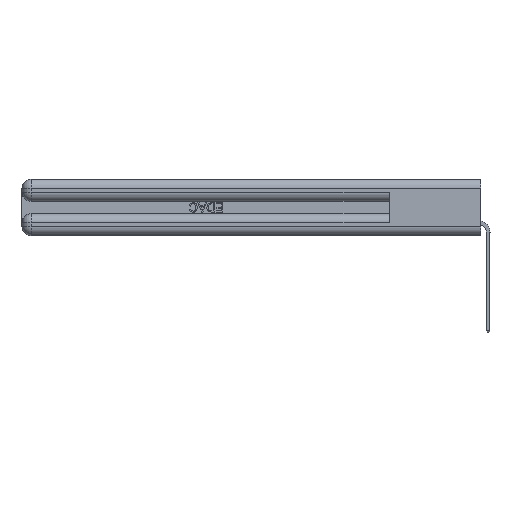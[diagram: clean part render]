
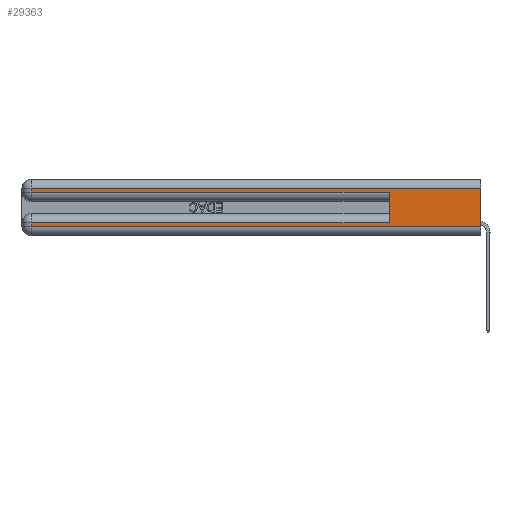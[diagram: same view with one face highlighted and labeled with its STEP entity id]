
A CAD part, left-side view. The second image highlights one B-rep face of the part: STEP entity #29363.
In plain terms, the highlighted planar face has unit normal (-1, 0, 0).
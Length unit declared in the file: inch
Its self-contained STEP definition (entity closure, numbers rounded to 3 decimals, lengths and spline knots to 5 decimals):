
#166 = DIRECTION ( 'NONE',  ( 0., 0., -1. ) ) ;
#222 = LINE ( 'NONE', #45272, #41382 ) ;
#773 = VECTOR ( 'NONE', #12997, 39.37008 ) ;
#2740 = EDGE_CURVE ( 'NONE', #19187, #14937, #31027, .T. ) ;
#3002 = EDGE_CURVE ( 'NONE', #6800, #37863, #222, .T. ) ;
#4448 = EDGE_CURVE ( 'NONE', #21822, #43918, #17563, .T. ) ;
#5373 = CARTESIAN_POINT ( 'NONE',  ( 0., 0., 0.31 ) ) ;
#5494 = PLANE ( 'NONE',  #32979 ) ;
#6591 = EDGE_CURVE ( 'NONE', #19187, #43918, #25633, .T. ) ;
#6682 = CARTESIAN_POINT ( 'NONE',  ( 0., 0.6, 0.145 ) ) ;
#6800 = VERTEX_POINT ( 'NONE', #9435 ) ;
#7109 = VECTOR ( 'NONE', #36315, 39.37008 ) ;
#7800 = VERTEX_POINT ( 'NONE', #29894 ) ;
#8801 = CARTESIAN_POINT ( 'NONE',  ( 0., 0., 0.37 ) ) ;
#9435 = CARTESIAN_POINT ( 'NONE',  ( 0., 2.94, 0.06 ) ) ;
#12997 = DIRECTION ( 'NONE',  ( 0., 0., -1. ) ) ;
#13910 = ORIENTED_EDGE ( 'NONE', *, *, #3002, .T. ) ;
#14516 = EDGE_CURVE ( 'NONE', #28528, #37863, #21750, .T. ) ;
#14787 = LINE ( 'NONE', #16875, #773 ) ;
#14937 = VERTEX_POINT ( 'NONE', #30757 ) ;
#15984 = VECTOR ( 'NONE', #29504, 39.37008 ) ;
#16369 = DIRECTION ( 'NONE',  ( 0., 0., -1. ) ) ;
#16875 = CARTESIAN_POINT ( 'NONE',  ( 0., 2.94, 0.37 ) ) ;
#17563 = LINE ( 'NONE', #45735, #30797 ) ;
#17865 = LINE ( 'NONE', #5373, #29418 ) ;
#19159 = DIRECTION ( 'NONE',  ( 0., 0., -1. ) ) ;
#19187 = VERTEX_POINT ( 'NONE', #41642 ) ;
#20234 = DIRECTION ( 'NONE',  ( 1., 0., 0. ) ) ;
#20458 = ORIENTED_EDGE ( 'NONE', *, *, #2740, .T. ) ;
#21311 = EDGE_LOOP ( 'NONE', ( #30749, #28575, #43992, #37009, #43074, #20458, #42451, #13910 ) ) ;
#21750 = LINE ( 'NONE', #8801, #28090 ) ;
#21822 = VERTEX_POINT ( 'NONE', #27001 ) ;
#22966 = DIRECTION ( 'NONE',  ( 0., -1., 0. ) ) ;
#23132 = EDGE_CURVE ( 'NONE', #7800, #21822, #14787, .T. ) ;
#25364 = EDGE_CURVE ( 'NONE', #28528, #7800, #17865, .T. ) ;
#25633 = LINE ( 'NONE', #6682, #7109 ) ;
#27001 = CARTESIAN_POINT ( 'NONE',  ( 0., 2.94, 0.285 ) ) ;
#28090 = VECTOR ( 'NONE', #19159, 39.37008 ) ;
#28445 = LINE ( 'NONE', #33699, #45779 ) ;
#28528 = VERTEX_POINT ( 'NONE', #40830 ) ;
#28575 = ORIENTED_EDGE ( 'NONE', *, *, #25364, .T. ) ;
#29363 = ADVANCED_FACE ( 'NONE', ( #40034 ), #5494, .F. ) ;
#29418 = VECTOR ( 'NONE', #46155, 39.37008 ) ;
#29504 = DIRECTION ( 'NONE',  ( 0., 1., 0. ) ) ;
#29894 = CARTESIAN_POINT ( 'NONE',  ( 0., 2.94, 0.31 ) ) ;
#30749 = ORIENTED_EDGE ( 'NONE', *, *, #14516, .F. ) ;
#30757 = CARTESIAN_POINT ( 'NONE',  ( 0., 2.94, 0.085 ) ) ;
#30797 = VECTOR ( 'NONE', #39087, 39.37008 ) ;
#31027 = LINE ( 'NONE', #33075, #15984 ) ;
#32979 = AXIS2_PLACEMENT_3D ( 'NONE', #34777, #20234, #16369 ) ;
#33075 = CARTESIAN_POINT ( 'NONE',  ( 0., 0., 0.085 ) ) ;
#33699 = CARTESIAN_POINT ( 'NONE',  ( 0., 2.94, 0.37 ) ) ;
#34777 = CARTESIAN_POINT ( 'NONE',  ( 0., 0., 0.37 ) ) ;
#36315 = DIRECTION ( 'NONE',  ( 0., 0., 1. ) ) ;
#37009 = ORIENTED_EDGE ( 'NONE', *, *, #4448, .T. ) ;
#37827 = CARTESIAN_POINT ( 'NONE',  ( 0., 0., 0.06 ) ) ;
#37863 = VERTEX_POINT ( 'NONE', #37827 ) ;
#39087 = DIRECTION ( 'NONE',  ( 0., -1., 0. ) ) ;
#40034 = FACE_OUTER_BOUND ( 'NONE', #21311, .T. ) ;
#40830 = CARTESIAN_POINT ( 'NONE',  ( 0., 0., 0.31 ) ) ;
#41382 = VECTOR ( 'NONE', #22966, 39.37008 ) ;
#41642 = CARTESIAN_POINT ( 'NONE',  ( 0., 0.6, 0.085 ) ) ;
#42451 = ORIENTED_EDGE ( 'NONE', *, *, #47200, .T. ) ;
#43074 = ORIENTED_EDGE ( 'NONE', *, *, #6591, .F. ) ;
#43918 = VERTEX_POINT ( 'NONE', #47215 ) ;
#43992 = ORIENTED_EDGE ( 'NONE', *, *, #23132, .T. ) ;
#45272 = CARTESIAN_POINT ( 'NONE',  ( 0., 0., 0.06 ) ) ;
#45735 = CARTESIAN_POINT ( 'NONE',  ( 0., 0., 0.285 ) ) ;
#45779 = VECTOR ( 'NONE', #166, 39.37008 ) ;
#46155 = DIRECTION ( 'NONE',  ( 0., 1., 0. ) ) ;
#47200 = EDGE_CURVE ( 'NONE', #14937, #6800, #28445, .T. ) ;
#47215 = CARTESIAN_POINT ( 'NONE',  ( 0., 0.6, 0.285 ) ) ;
